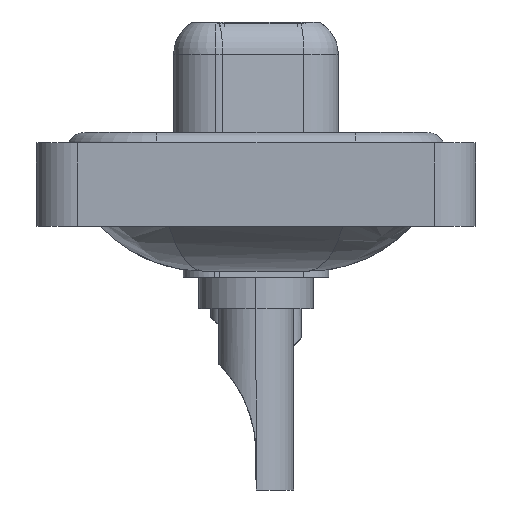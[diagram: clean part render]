
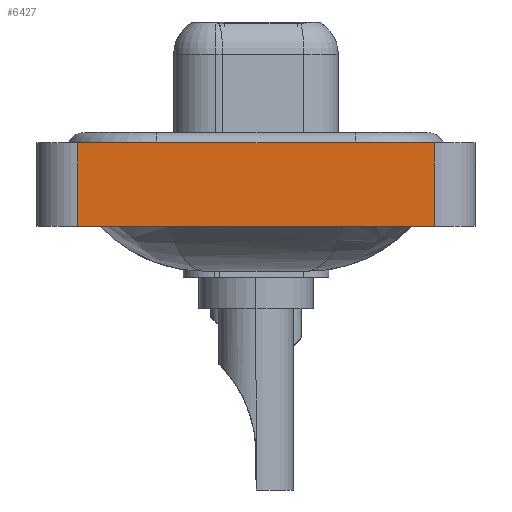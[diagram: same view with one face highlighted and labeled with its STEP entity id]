
A CAD part, left-side view. The second image highlights one B-rep face of the part: STEP entity #6427.
In plain terms, the highlighted planar face has unit normal (-1, 0, 0).
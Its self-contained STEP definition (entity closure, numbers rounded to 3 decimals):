
#1474 = VECTOR ( 'NONE', #11827, 1000. ) ;
#2092 = CARTESIAN_POINT ( 'NONE',  ( -7.35, -8.55, 0.4 ) ) ;
#2567 = VERTEX_POINT ( 'NONE', #14960 ) ;
#2903 = AXIS2_PLACEMENT_3D ( 'NONE', #10400, #8314, #19076 ) ;
#3496 = PLANE ( 'NONE',  #2903 ) ;
#3525 = VECTOR ( 'NONE', #11379, 1000. ) ;
#4683 = ORIENTED_EDGE ( 'NONE', *, *, #6482, .F. ) ;
#4772 = EDGE_CURVE ( 'NONE', #2567, #5273, #9833, .T. ) ;
#5273 = VERTEX_POINT ( 'NONE', #7944 ) ;
#6427 = ADVANCED_FACE ( 'NONE', ( #15930 ), #3496, .T. ) ;
#6482 = EDGE_CURVE ( 'NONE', #5273, #8720, #10871, .T. ) ;
#7944 = CARTESIAN_POINT ( 'NONE',  ( -7.35, 8.55, 0.4 ) ) ;
#8314 = DIRECTION ( 'NONE',  ( -1., 0., 0. ) ) ;
#8720 = VERTEX_POINT ( 'NONE', #22777 ) ;
#8779 = ORIENTED_EDGE ( 'NONE', *, *, #4772, .F. ) ;
#9334 = DIRECTION ( 'NONE',  ( 0., -1., 0. ) ) ;
#9447 = DIRECTION ( 'NONE',  ( 0., 0., 1. ) ) ;
#9784 = CARTESIAN_POINT ( 'NONE',  ( -7.35, -8.55, -3.6 ) ) ;
#9833 = LINE ( 'NONE', #22032, #1474 ) ;
#10400 = CARTESIAN_POINT ( 'NONE',  ( -7.35, -8.55, -3.6 ) ) ;
#10871 = LINE ( 'NONE', #2092, #15623 ) ;
#11379 = DIRECTION ( 'NONE',  ( 0., -1., 0. ) ) ;
#11827 = DIRECTION ( 'NONE',  ( 0., 0., 1. ) ) ;
#12904 = LINE ( 'NONE', #18415, #3525 ) ;
#14046 = EDGE_CURVE ( 'NONE', #16377, #8720, #16618, .T. ) ;
#14657 = EDGE_LOOP ( 'NONE', ( #21961, #4683, #8779, #21268 ) ) ;
#14960 = CARTESIAN_POINT ( 'NONE',  ( -7.35, 8.55, -3.6 ) ) ;
#15623 = VECTOR ( 'NONE', #9334, 1000. ) ;
#15930 = FACE_OUTER_BOUND ( 'NONE', #14657, .T. ) ;
#16120 = VECTOR ( 'NONE', #9447, 1000. ) ;
#16377 = VERTEX_POINT ( 'NONE', #20182 ) ;
#16618 = LINE ( 'NONE', #9784, #16120 ) ;
#18415 = CARTESIAN_POINT ( 'NONE',  ( -7.35, -8.55, -3.6 ) ) ;
#19076 = DIRECTION ( 'NONE',  ( 0., 0., 1. ) ) ;
#19704 = EDGE_CURVE ( 'NONE', #2567, #16377, #12904, .T. ) ;
#20182 = CARTESIAN_POINT ( 'NONE',  ( -7.35, -8.55, -3.6 ) ) ;
#21268 = ORIENTED_EDGE ( 'NONE', *, *, #19704, .T. ) ;
#21961 = ORIENTED_EDGE ( 'NONE', *, *, #14046, .T. ) ;
#22032 = CARTESIAN_POINT ( 'NONE',  ( -7.35, 8.55, -3.6 ) ) ;
#22777 = CARTESIAN_POINT ( 'NONE',  ( -7.35, -8.55, 0.4 ) ) ;
